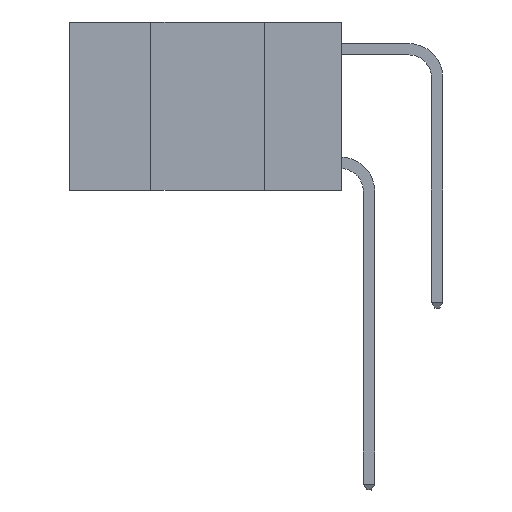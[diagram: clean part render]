
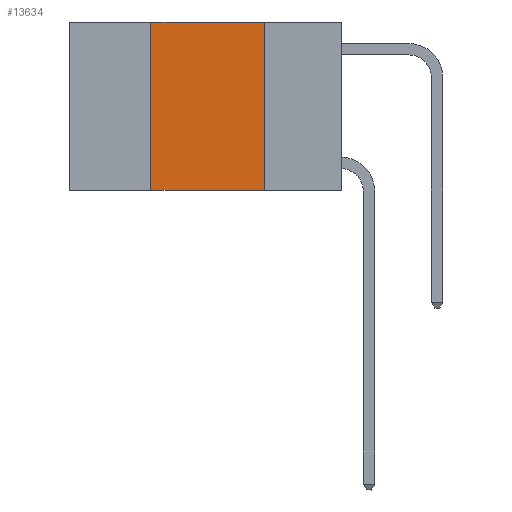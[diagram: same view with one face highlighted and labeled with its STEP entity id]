
A CAD part, left-side view. The second image highlights one B-rep face of the part: STEP entity #13634.
In plain terms, the highlighted planar face has unit normal (-1, 0, 0).
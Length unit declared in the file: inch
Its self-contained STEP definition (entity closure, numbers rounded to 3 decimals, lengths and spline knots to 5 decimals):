
#625 = EDGE_LOOP ( 'NONE', ( #2807, #14596, #24270, #19424 ) ) ;
#2134 = VECTOR ( 'NONE', #7350, 39.37008 ) ;
#2725 = CARTESIAN_POINT ( 'NONE',  ( 0., 0.17, 0. ) ) ;
#2807 = ORIENTED_EDGE ( 'NONE', *, *, #21696, .F. ) ;
#3331 = VERTEX_POINT ( 'NONE', #2725 ) ;
#3530 = CARTESIAN_POINT ( 'NONE',  ( 0., 0.17, 0. ) ) ;
#4153 = VERTEX_POINT ( 'NONE', #22377 ) ;
#6106 = VECTOR ( 'NONE', #15535, 39.37008 ) ;
#6988 = DIRECTION ( 'NONE',  ( 0., -1., 0. ) ) ;
#7350 = DIRECTION ( 'NONE',  ( 0., 0., 1. ) ) ;
#8907 = VECTOR ( 'NONE', #9832, 39.37008 ) ;
#9648 = VECTOR ( 'NONE', #6988, 39.37008 ) ;
#9832 = DIRECTION ( 'NONE',  ( 0., 0., -1. ) ) ;
#10057 = PLANE ( 'NONE',  #13948 ) ;
#10299 = LINE ( 'NONE', #11182, #9648 ) ;
#11182 = CARTESIAN_POINT ( 'NONE',  ( 0., 0.6, 0. ) ) ;
#11945 = EDGE_CURVE ( 'NONE', #4153, #17343, #22737, .T. ) ;
#12151 = DIRECTION ( 'NONE',  ( 1., 0., 0. ) ) ;
#13634 = ADVANCED_FACE ( 'NONE', ( #20347 ), #10057, .F. ) ;
#13948 = AXIS2_PLACEMENT_3D ( 'NONE', #22525, #12151, #26653 ) ;
#14481 = LINE ( 'NONE', #3530, #8907 ) ;
#14596 = ORIENTED_EDGE ( 'NONE', *, *, #24348, .F. ) ;
#15535 = DIRECTION ( 'NONE',  ( 0., -1., 0. ) ) ;
#15678 = CARTESIAN_POINT ( 'NONE',  ( 0., 0.42, 0. ) ) ;
#16175 = CARTESIAN_POINT ( 'NONE',  ( 0., 0.42, 0. ) ) ;
#17343 = VERTEX_POINT ( 'NONE', #22813 ) ;
#19424 = ORIENTED_EDGE ( 'NONE', *, *, #11945, .T. ) ;
#20347 = FACE_OUTER_BOUND ( 'NONE', #625, .T. ) ;
#21023 = VERTEX_POINT ( 'NONE', #16175 ) ;
#21685 = CARTESIAN_POINT ( 'NONE',  ( 0., 0.6, -0.37 ) ) ;
#21696 = EDGE_CURVE ( 'NONE', #3331, #17343, #14481, .T. ) ;
#22377 = CARTESIAN_POINT ( 'NONE',  ( 0., 0.42, -0.37 ) ) ;
#22525 = CARTESIAN_POINT ( 'NONE',  ( 0., 0.6, 0. ) ) ;
#22737 = LINE ( 'NONE', #21685, #6106 ) ;
#22813 = CARTESIAN_POINT ( 'NONE',  ( 0., 0.17, -0.37 ) ) ;
#24258 = LINE ( 'NONE', #15678, #2134 ) ;
#24270 = ORIENTED_EDGE ( 'NONE', *, *, #24452, .F. ) ;
#24348 = EDGE_CURVE ( 'NONE', #21023, #3331, #10299, .T. ) ;
#24452 = EDGE_CURVE ( 'NONE', #4153, #21023, #24258, .T. ) ;
#26653 = DIRECTION ( 'NONE',  ( 0., 0., -1. ) ) ;
